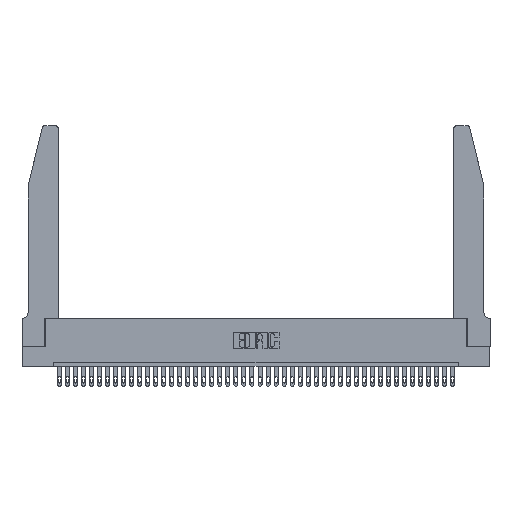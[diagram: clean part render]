
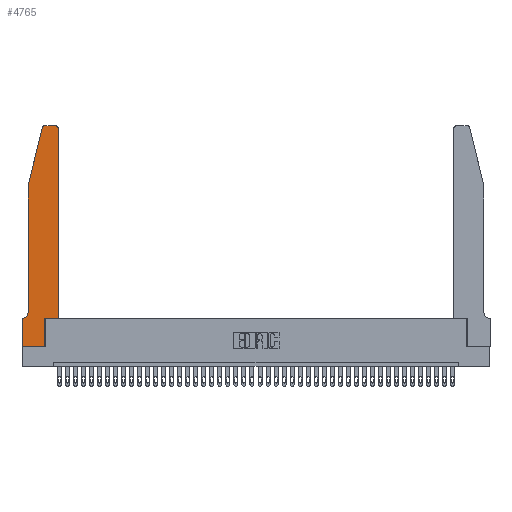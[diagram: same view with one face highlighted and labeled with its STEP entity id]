
A CAD part, top view. The second image highlights one B-rep face of the part: STEP entity #4765.
In plain terms, the highlighted planar face has unit normal (0, 0, 1).
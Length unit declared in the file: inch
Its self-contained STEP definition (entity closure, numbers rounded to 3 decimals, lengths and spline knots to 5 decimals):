
#432 = ORIENTED_EDGE ( 'NONE', *, *, #23222, .T. ) ;
#1067 = CARTESIAN_POINT ( 'NONE',  ( 0.2865, 0.35, 0.37 ) ) ;
#1309 = ORIENTED_EDGE ( 'NONE', *, *, #23379, .T. ) ;
#1595 = VECTOR ( 'NONE', #26877, 39.37008 ) ;
#1607 = CARTESIAN_POINT ( 'NONE',  ( 0.0755, 2., 0.37 ) ) ;
#1787 = DIRECTION ( 'NONE',  ( 0., 0., 1. ) ) ;
#2929 = VERTEX_POINT ( 'NONE', #32137 ) ;
#3248 = VERTEX_POINT ( 'NONE', #24264 ) ;
#3946 = DIRECTION ( 'NONE',  ( -1., 0., 0. ) ) ;
#4479 = EDGE_CURVE ( 'NONE', #40647, #40271, #21192, .T. ) ;
#4512 = CARTESIAN_POINT ( 'NONE',  ( 0.0755, 2., 0.37 ) ) ;
#4765 = ADVANCED_FACE ( 'NONE', ( #7267 ), #29388, .T. ) ;
#5741 = AXIS2_PLACEMENT_3D ( 'NONE', #35221, #39250, #20158 ) ;
#6100 = ORIENTED_EDGE ( 'NONE', *, *, #11591, .T. ) ;
#6589 = LINE ( 'NONE', #1607, #1595 ) ;
#6905 = DIRECTION ( 'NONE',  ( 0., 0., 1. ) ) ;
#7267 = FACE_OUTER_BOUND ( 'NONE', #28551, .T. ) ;
#7555 = VERTEX_POINT ( 'NONE', #18597 ) ;
#7689 = LINE ( 'NONE', #39436, #21083 ) ;
#9457 = CARTESIAN_POINT ( 'NONE',  ( 0.4505, 2.72, 0.37 ) ) ;
#10159 = CARTESIAN_POINT ( 'NONE',  ( 0.0055, 0.42, 0.37 ) ) ;
#11422 = EDGE_CURVE ( 'NONE', #2929, #3248, #29135, .T. ) ;
#11568 = LINE ( 'NONE', #32703, #34924 ) ;
#11591 = EDGE_CURVE ( 'NONE', #35249, #2929, #31637, .T. ) ;
#13313 = CIRCLE ( 'NONE', #40471, 0.03 ) ;
#13319 = DIRECTION ( 'NONE',  ( 0., 0., -1. ) ) ;
#13322 = AXIS2_PLACEMENT_3D ( 'NONE', #35228, #6905, #32307 ) ;
#13419 = VERTEX_POINT ( 'NONE', #27603 ) ;
#13752 = VECTOR ( 'NONE', #17487, 39.37008 ) ;
#14141 = ORIENTED_EDGE ( 'NONE', *, *, #22442, .T. ) ;
#14143 = DIRECTION ( 'NONE',  ( 0., -1., 0. ) ) ;
#15443 = DIRECTION ( 'NONE',  ( 0., 1., 0. ) ) ;
#15640 = CARTESIAN_POINT ( 'NONE',  ( 0.4505, 0.35, 0.37 ) ) ;
#16507 = VECTOR ( 'NONE', #15443, 39.37008 ) ;
#16867 = ORIENTED_EDGE ( 'NONE', *, *, #32823, .T. ) ;
#17487 = DIRECTION ( 'NONE',  ( 0., 1., 0. ) ) ;
#17682 = VERTEX_POINT ( 'NONE', #38788 ) ;
#18153 = ORIENTED_EDGE ( 'NONE', *, *, #4479, .T. ) ;
#18531 = EDGE_CURVE ( 'NONE', #40271, #13419, #40825, .T. ) ;
#18597 = CARTESIAN_POINT ( 'NONE',  ( 0., 0.35, 0.37 ) ) ;
#20158 = DIRECTION ( 'NONE',  ( 1., 0., 0. ) ) ;
#21083 = VECTOR ( 'NONE', #26788, 39.37008 ) ;
#21192 = CIRCLE ( 'NONE', #13322, 0.03 ) ;
#21443 = EDGE_CURVE ( 'NONE', #22150, #17682, #7689, .T. ) ;
#22150 = VERTEX_POINT ( 'NONE', #26055 ) ;
#22442 = EDGE_CURVE ( 'NONE', #7555, #22150, #32973, .T. ) ;
#23222 = EDGE_CURVE ( 'NONE', #26612, #28815, #11568, .T. ) ;
#23379 = EDGE_CURVE ( 'NONE', #35361, #35249, #6589, .T. ) ;
#23477 = VECTOR ( 'NONE', #32843, 39.37008 ) ;
#23697 = LINE ( 'NONE', #26989, #13752 ) ;
#23943 = DIRECTION ( 'NONE',  ( 1., 0., 0. ) ) ;
#24264 = CARTESIAN_POINT ( 'NONE',  ( 0.0055, 0.35, 0.37 ) ) ;
#24594 = ORIENTED_EDGE ( 'NONE', *, *, #21443, .T. ) ;
#25057 = CARTESIAN_POINT ( 'NONE',  ( 0.2605, 2.75, 0.37 ) ) ;
#26055 = CARTESIAN_POINT ( 'NONE',  ( 0., 0., 0.37 ) ) ;
#26612 = VERTEX_POINT ( 'NONE', #1067 ) ;
#26788 = DIRECTION ( 'NONE',  ( 1., 0., 0. ) ) ;
#26877 = DIRECTION ( 'NONE',  ( -0.239, -0.971, 0. ) ) ;
#26989 = CARTESIAN_POINT ( 'NONE',  ( 0.2865, 0.35, 0.37 ) ) ;
#27531 = LINE ( 'NONE', #40694, #39403 ) ;
#27603 = CARTESIAN_POINT ( 'NONE',  ( 0.284, 2.75, 0.37 ) ) ;
#28551 = EDGE_LOOP ( 'NONE', ( #38613, #16867, #1309, #6100, #37491, #38547, #14141, #24594, #29726, #432, #33583, #18153 ) ) ;
#28815 = VERTEX_POINT ( 'NONE', #15640 ) ;
#29135 = CIRCLE ( 'NONE', #40480, 0.07 ) ;
#29388 = PLANE ( 'NONE',  #5741 ) ;
#29726 = ORIENTED_EDGE ( 'NONE', *, *, #33503, .T. ) ;
#30088 = EDGE_CURVE ( 'NONE', #3248, #7555, #27531, .T. ) ;
#30811 = DIRECTION ( 'NONE',  ( -1., 0., 0. ) ) ;
#31174 = VECTOR ( 'NONE', #14143, 39.37008 ) ;
#31637 = LINE ( 'NONE', #32958, #31174 ) ;
#32137 = CARTESIAN_POINT ( 'NONE',  ( 0.0755, 0.42, 0.37 ) ) ;
#32277 = VECTOR ( 'NONE', #38030, 39.37008 ) ;
#32307 = DIRECTION ( 'NONE',  ( 1., 0., 0. ) ) ;
#32703 = CARTESIAN_POINT ( 'NONE',  ( 0.4505, 0.35, 0.37 ) ) ;
#32823 = EDGE_CURVE ( 'NONE', #13419, #35361, #13313, .T. ) ;
#32836 = DIRECTION ( 'NONE',  ( 1., 0., 0. ) ) ;
#32843 = DIRECTION ( 'NONE',  ( 0., -1., 0. ) ) ;
#32958 = CARTESIAN_POINT ( 'NONE',  ( 0.0755, 2., 0.37 ) ) ;
#32973 = LINE ( 'NONE', #38965, #23477 ) ;
#33442 = CARTESIAN_POINT ( 'NONE',  ( 0.284, 2.72, 0.37 ) ) ;
#33503 = EDGE_CURVE ( 'NONE', #17682, #26612, #23697, .T. ) ;
#33583 = ORIENTED_EDGE ( 'NONE', *, *, #39889, .T. ) ;
#34394 = CARTESIAN_POINT ( 'NONE',  ( 0.4505, 0.35, 0.37 ) ) ;
#34924 = VECTOR ( 'NONE', #32836, 39.37008 ) ;
#35221 = CARTESIAN_POINT ( 'NONE',  ( 0., 0.35, 0.37 ) ) ;
#35228 = CARTESIAN_POINT ( 'NONE',  ( 0.4205, 2.72, 0.37 ) ) ;
#35249 = VERTEX_POINT ( 'NONE', #4512 ) ;
#35361 = VERTEX_POINT ( 'NONE', #37301 ) ;
#35849 = CARTESIAN_POINT ( 'NONE',  ( 0.4205, 2.75, 0.37 ) ) ;
#37301 = CARTESIAN_POINT ( 'NONE',  ( 0.25487, 2.72718, 0.37 ) ) ;
#37491 = ORIENTED_EDGE ( 'NONE', *, *, #11422, .T. ) ;
#37514 = LINE ( 'NONE', #34394, #16507 ) ;
#38030 = DIRECTION ( 'NONE',  ( -1., 0., 0. ) ) ;
#38547 = ORIENTED_EDGE ( 'NONE', *, *, #30088, .T. ) ;
#38613 = ORIENTED_EDGE ( 'NONE', *, *, #18531, .T. ) ;
#38788 = CARTESIAN_POINT ( 'NONE',  ( 0.2865, 0., 0.37 ) ) ;
#38965 = CARTESIAN_POINT ( 'NONE',  ( 0., 0., 0.37 ) ) ;
#39250 = DIRECTION ( 'NONE',  ( 0., 0., 1. ) ) ;
#39403 = VECTOR ( 'NONE', #30811, 39.37008 ) ;
#39436 = CARTESIAN_POINT ( 'NONE',  ( 0., 0., 0.37 ) ) ;
#39889 = EDGE_CURVE ( 'NONE', #28815, #40647, #37514, .T. ) ;
#40271 = VERTEX_POINT ( 'NONE', #35849 ) ;
#40471 = AXIS2_PLACEMENT_3D ( 'NONE', #33442, #1787, #23943 ) ;
#40480 = AXIS2_PLACEMENT_3D ( 'NONE', #10159, #13319, #3946 ) ;
#40647 = VERTEX_POINT ( 'NONE', #9457 ) ;
#40694 = CARTESIAN_POINT ( 'NONE',  ( 0.0755, 0.35, 0.37 ) ) ;
#40825 = LINE ( 'NONE', #25057, #32277 ) ;
